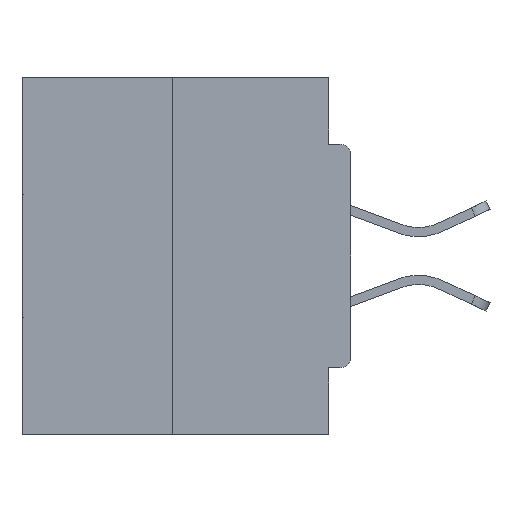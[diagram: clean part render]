
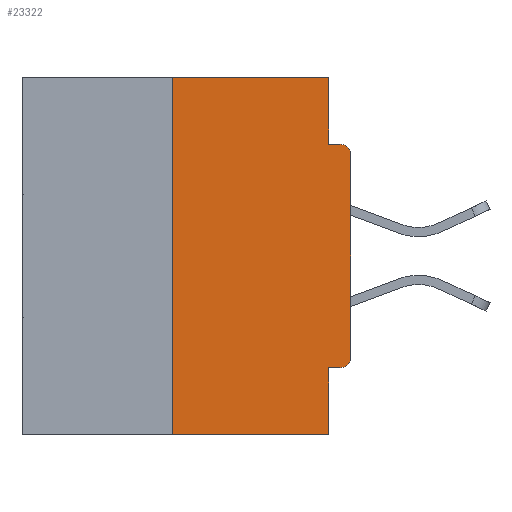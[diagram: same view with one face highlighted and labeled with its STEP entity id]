
A CAD part, left-side view. The second image highlights one B-rep face of the part: STEP entity #23322.
In plain terms, the highlighted planar face has unit normal (-1, 0, 0).
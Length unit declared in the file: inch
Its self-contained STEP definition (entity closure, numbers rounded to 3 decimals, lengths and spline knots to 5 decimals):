
#794 = VERTEX_POINT ( 'NONE', #13840 ) ;
#1707 = ORIENTED_EDGE ( 'NONE', *, *, #37285, .T. ) ;
#2790 = VERTEX_POINT ( 'NONE', #8837 ) ;
#2909 = VECTOR ( 'NONE', #15442, 39.37008 ) ;
#3136 = DIRECTION ( 'NONE',  ( 0., 0., -1. ) ) ;
#3270 = CARTESIAN_POINT ( 'NONE',  ( 0., 0.25, 0. ) ) ;
#3321 = EDGE_CURVE ( 'NONE', #9283, #31756, #28247, .T. ) ;
#3325 = VECTOR ( 'NONE', #37018, 39.37008 ) ;
#3413 = LINE ( 'NONE', #11716, #11079 ) ;
#3833 = DIRECTION ( 'NONE',  ( -1., 0., 0. ) ) ;
#4659 = ORIENTED_EDGE ( 'NONE', *, *, #29144, .T. ) ;
#5483 = CARTESIAN_POINT ( 'NONE',  ( 0., 0., -0.0935 ) ) ;
#5858 = DIRECTION ( 'NONE',  ( 1., 0., 0. ) ) ;
#6552 = AXIS2_PLACEMENT_3D ( 'NONE', #36704, #33602, #39278 ) ;
#7308 = LINE ( 'NONE', #5483, #39371 ) ;
#7468 = DIRECTION ( 'NONE',  ( 0., 0., 1. ) ) ;
#7552 = CARTESIAN_POINT ( 'NONE',  ( 0., 0.031, -0.5 ) ) ;
#8837 = CARTESIAN_POINT ( 'NONE',  ( 0., 0., -0.1085 ) ) ;
#9283 = VERTEX_POINT ( 'NONE', #11510 ) ;
#9332 = CARTESIAN_POINT ( 'NONE',  ( 0., 0.46, 0. ) ) ;
#9812 = VECTOR ( 'NONE', #30378, 39.37008 ) ;
#10007 = ORIENTED_EDGE ( 'NONE', *, *, #20823, .F. ) ;
#10794 = CARTESIAN_POINT ( 'NONE',  ( 0., 0.031, -0.4065 ) ) ;
#11079 = VECTOR ( 'NONE', #33332, 39.37008 ) ;
#11510 = CARTESIAN_POINT ( 'NONE',  ( 0., 0.015, -0.4065 ) ) ;
#11716 = CARTESIAN_POINT ( 'NONE',  ( 0., 0.031, -0.5 ) ) ;
#12202 = EDGE_CURVE ( 'NONE', #9283, #24257, #18867, .T. ) ;
#13532 = AXIS2_PLACEMENT_3D ( 'NONE', #9332, #5858, #18303 ) ;
#13840 = CARTESIAN_POINT ( 'NONE',  ( 0., 0.25, -0.5 ) ) ;
#14821 = CARTESIAN_POINT ( 'NONE',  ( 0., 0.46, 0. ) ) ;
#15001 = CARTESIAN_POINT ( 'NONE',  ( 0., 0.031, 0. ) ) ;
#15310 = CARTESIAN_POINT ( 'NONE',  ( 0., 0., -0.4065 ) ) ;
#15442 = DIRECTION ( 'NONE',  ( 0., 1., 0. ) ) ;
#16825 = LINE ( 'NONE', #15001, #29044 ) ;
#17774 = VERTEX_POINT ( 'NONE', #7552 ) ;
#18104 = LINE ( 'NONE', #36579, #9812 ) ;
#18303 = DIRECTION ( 'NONE',  ( 0., 0., -1. ) ) ;
#18867 = LINE ( 'NONE', #15310, #2909 ) ;
#18958 = ORIENTED_EDGE ( 'NONE', *, *, #12202, .F. ) ;
#19667 = VECTOR ( 'NONE', #23219, 39.37008 ) ;
#19670 = LINE ( 'NONE', #28963, #22617 ) ;
#20184 = ORIENTED_EDGE ( 'NONE', *, *, #20806, .F. ) ;
#20208 = ORIENTED_EDGE ( 'NONE', *, *, #3321, .T. ) ;
#20783 = ORIENTED_EDGE ( 'NONE', *, *, #21249, .F. ) ;
#20806 = EDGE_CURVE ( 'NONE', #37012, #28890, #16825, .T. ) ;
#20823 = EDGE_CURVE ( 'NONE', #794, #24109, #36302, .T. ) ;
#20959 = FACE_OUTER_BOUND ( 'NONE', #24580, .T. ) ;
#21249 = EDGE_CURVE ( 'NONE', #24109, #37012, #21635, .T. ) ;
#21326 = DIRECTION ( 'NONE',  ( 0., -1., 0. ) ) ;
#21574 = PLANE ( 'NONE',  #13532 ) ;
#21635 = LINE ( 'NONE', #14821, #19667 ) ;
#21963 = AXIS2_PLACEMENT_3D ( 'NONE', #37993, #3833, #25815 ) ;
#22505 = CARTESIAN_POINT ( 'NONE',  ( 0., 0.25, 0. ) ) ;
#22617 = VECTOR ( 'NONE', #7468, 39.37008 ) ;
#23219 = DIRECTION ( 'NONE',  ( 0., -1., 0. ) ) ;
#23322 = ADVANCED_FACE ( 'NONE', ( #20959 ), #21574, .F. ) ;
#24023 = EDGE_CURVE ( 'NONE', #28890, #38392, #7308, .T. ) ;
#24109 = VERTEX_POINT ( 'NONE', #22505 ) ;
#24257 = VERTEX_POINT ( 'NONE', #10794 ) ;
#24580 = EDGE_LOOP ( 'NONE', ( #20783, #10007, #26694, #35615, #18958, #20208, #1707, #4659, #38094, #20184 ) ) ;
#25815 = DIRECTION ( 'NONE',  ( 0., 0., -1. ) ) ;
#26694 = ORIENTED_EDGE ( 'NONE', *, *, #39192, .T. ) ;
#26777 = CIRCLE ( 'NONE', #6552, 0.015 ) ;
#27861 = CARTESIAN_POINT ( 'NONE',  ( 0., 0.031, -0.0935 ) ) ;
#28053 = CARTESIAN_POINT ( 'NONE',  ( 0., 0., -0.3915 ) ) ;
#28247 = CIRCLE ( 'NONE', #21963, 0.015 ) ;
#28890 = VERTEX_POINT ( 'NONE', #27861 ) ;
#28963 = CARTESIAN_POINT ( 'NONE',  ( 0., 0., 0. ) ) ;
#29044 = VECTOR ( 'NONE', #3136, 39.37008 ) ;
#29144 = EDGE_CURVE ( 'NONE', #2790, #38392, #26777, .T. ) ;
#30213 = EDGE_CURVE ( 'NONE', #24257, #17774, #3413, .T. ) ;
#30378 = DIRECTION ( 'NONE',  ( 0., -1., 0. ) ) ;
#30766 = CARTESIAN_POINT ( 'NONE',  ( 0., 0.031, 0. ) ) ;
#31756 = VERTEX_POINT ( 'NONE', #28053 ) ;
#33332 = DIRECTION ( 'NONE',  ( 0., 0., -1. ) ) ;
#33602 = DIRECTION ( 'NONE',  ( -1., 0., 0. ) ) ;
#35615 = ORIENTED_EDGE ( 'NONE', *, *, #30213, .F. ) ;
#36302 = LINE ( 'NONE', #3270, #3325 ) ;
#36579 = CARTESIAN_POINT ( 'NONE',  ( 0., 0.46, -0.5 ) ) ;
#36704 = CARTESIAN_POINT ( 'NONE',  ( 0., 0.015, -0.1085 ) ) ;
#37012 = VERTEX_POINT ( 'NONE', #30766 ) ;
#37018 = DIRECTION ( 'NONE',  ( 0., 0., 1. ) ) ;
#37285 = EDGE_CURVE ( 'NONE', #31756, #2790, #19670, .T. ) ;
#37993 = CARTESIAN_POINT ( 'NONE',  ( 0., 0.015, -0.3915 ) ) ;
#38094 = ORIENTED_EDGE ( 'NONE', *, *, #24023, .F. ) ;
#38392 = VERTEX_POINT ( 'NONE', #38782 ) ;
#38782 = CARTESIAN_POINT ( 'NONE',  ( 0., 0.015, -0.0935 ) ) ;
#39192 = EDGE_CURVE ( 'NONE', #794, #17774, #18104, .T. ) ;
#39278 = DIRECTION ( 'NONE',  ( 0., 0., -1. ) ) ;
#39371 = VECTOR ( 'NONE', #21326, 39.37008 ) ;
